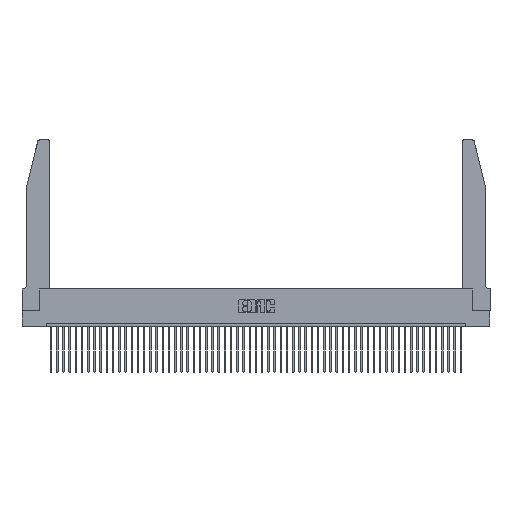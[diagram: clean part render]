
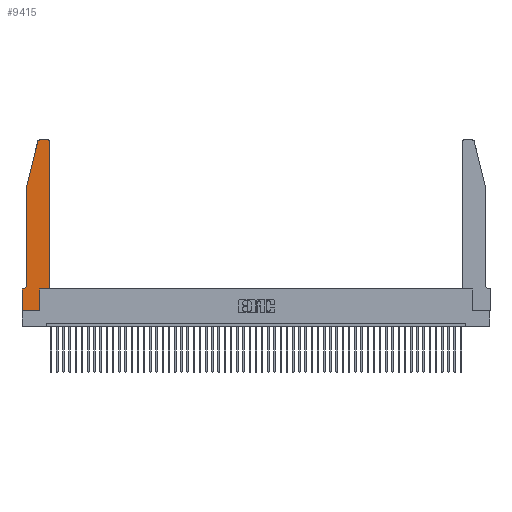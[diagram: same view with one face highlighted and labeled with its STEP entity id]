
A CAD part, top view. The second image highlights one B-rep face of the part: STEP entity #9415.
In plain terms, the highlighted planar face has unit normal (0, 0, 1).
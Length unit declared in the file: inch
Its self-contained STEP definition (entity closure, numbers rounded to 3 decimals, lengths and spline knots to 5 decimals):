
#374 = LINE ( 'NONE', #10518, #41643 ) ;
#1106 = VECTOR ( 'NONE', #31325, 39.37008 ) ;
#1204 = LINE ( 'NONE', #6719, #50765 ) ;
#2429 = CARTESIAN_POINT ( 'NONE',  ( 0.0755, 2., 0.37 ) ) ;
#2513 = ORIENTED_EDGE ( 'NONE', *, *, #3123, .T. ) ;
#2647 = EDGE_CURVE ( 'NONE', #16908, #18921, #16390, .T. ) ;
#2677 = EDGE_CURVE ( 'NONE', #35135, #7673, #44608, .T. ) ;
#3123 = EDGE_CURVE ( 'NONE', #8637, #47665, #18210, .T. ) ;
#3977 = CARTESIAN_POINT ( 'NONE',  ( 0., 0., 0.37 ) ) ;
#4345 = VERTEX_POINT ( 'NONE', #3977 ) ;
#4690 = EDGE_CURVE ( 'NONE', #18921, #37646, #39350, .T. ) ;
#5635 = CARTESIAN_POINT ( 'NONE',  ( 0.4505, 0.35, 0.37 ) ) ;
#5920 = EDGE_CURVE ( 'NONE', #7673, #25662, #12362, .T. ) ;
#6370 = DIRECTION ( 'NONE',  ( -1., 0., 0. ) ) ;
#6393 = EDGE_CURVE ( 'NONE', #35458, #16908, #32844, .T. ) ;
#6719 = CARTESIAN_POINT ( 'NONE',  ( 0.2605, 2.75, 0.37 ) ) ;
#7445 = PLANE ( 'NONE',  #38423 ) ;
#7526 = ORIENTED_EDGE ( 'NONE', *, *, #4690, .T. ) ;
#7673 = VERTEX_POINT ( 'NONE', #41694 ) ;
#7731 = VECTOR ( 'NONE', #43276, 39.37008 ) ;
#7817 = DIRECTION ( 'NONE',  ( 1., 0., 0. ) ) ;
#8637 = VERTEX_POINT ( 'NONE', #9405 ) ;
#9405 = CARTESIAN_POINT ( 'NONE',  ( 0.4505, 2.72, 0.37 ) ) ;
#9415 = ADVANCED_FACE ( 'NONE', ( #12563 ), #7445, .T. ) ;
#10518 = CARTESIAN_POINT ( 'NONE',  ( 0.0755, 0.35, 0.37 ) ) ;
#10722 = DIRECTION ( 'NONE',  ( 1., 0., 0. ) ) ;
#12362 = LINE ( 'NONE', #39153, #47496 ) ;
#12563 = FACE_OUTER_BOUND ( 'NONE', #18466, .T. ) ;
#13624 = CARTESIAN_POINT ( 'NONE',  ( 0.0755, 0.42, 0.37 ) ) ;
#14068 = AXIS2_PLACEMENT_3D ( 'NONE', #38728, #31158, #18724 ) ;
#14349 = DIRECTION ( 'NONE',  ( -1., 0., 0. ) ) ;
#14564 = CARTESIAN_POINT ( 'NONE',  ( 0., 0.35, 0.37 ) ) ;
#15141 = CARTESIAN_POINT ( 'NONE',  ( 0.284, 2.72, 0.37 ) ) ;
#15392 = VECTOR ( 'NONE', #33100, 39.37008 ) ;
#15919 = ORIENTED_EDGE ( 'NONE', *, *, #20522, .T. ) ;
#16390 = LINE ( 'NONE', #39221, #7731 ) ;
#16908 = VERTEX_POINT ( 'NONE', #48533 ) ;
#17867 = EDGE_CURVE ( 'NONE', #47665, #35458, #1204, .T. ) ;
#18210 = CIRCLE ( 'NONE', #14068, 0.03 ) ;
#18466 = EDGE_LOOP ( 'NONE', ( #30757, #20926, #44212, #7526, #37136, #26081, #39527, #15919, #37426, #43944, #51509, #2513 ) ) ;
#18724 = DIRECTION ( 'NONE',  ( 1., 0., 0. ) ) ;
#18921 = VERTEX_POINT ( 'NONE', #26406 ) ;
#19129 = DIRECTION ( 'NONE',  ( 1., 0., 0. ) ) ;
#19194 = CARTESIAN_POINT ( 'NONE',  ( 0.2865, 0., 0.37 ) ) ;
#19353 = VERTEX_POINT ( 'NONE', #50166 ) ;
#20522 = EDGE_CURVE ( 'NONE', #4345, #35135, #46096, .T. ) ;
#20926 = ORIENTED_EDGE ( 'NONE', *, *, #6393, .T. ) ;
#22070 = AXIS2_PLACEMENT_3D ( 'NONE', #39352, #30908, #39514 ) ;
#22544 = CARTESIAN_POINT ( 'NONE',  ( 0.4505, 0.35, 0.37 ) ) ;
#22667 = VECTOR ( 'NONE', #26216, 39.37008 ) ;
#23371 = VECTOR ( 'NONE', #35500, 39.37008 ) ;
#23710 = DIRECTION ( 'NONE',  ( 0., 0., 1. ) ) ;
#24046 = VECTOR ( 'NONE', #24860, 39.37008 ) ;
#24351 = VERTEX_POINT ( 'NONE', #49802 ) ;
#24860 = DIRECTION ( 'NONE',  ( 0., -1., 0. ) ) ;
#25662 = VERTEX_POINT ( 'NONE', #5635 ) ;
#26081 = ORIENTED_EDGE ( 'NONE', *, *, #37822, .T. ) ;
#26216 = DIRECTION ( 'NONE',  ( 0., 1., 0. ) ) ;
#26406 = CARTESIAN_POINT ( 'NONE',  ( 0.0755, 2., 0.37 ) ) ;
#29647 = CARTESIAN_POINT ( 'NONE',  ( 0., 0., 0.37 ) ) ;
#30581 = AXIS2_PLACEMENT_3D ( 'NONE', #15141, #23710, #7817 ) ;
#30757 = ORIENTED_EDGE ( 'NONE', *, *, #17867, .T. ) ;
#30908 = DIRECTION ( 'NONE',  ( 0., 0., -1. ) ) ;
#31140 = DIRECTION ( 'NONE',  ( 0., 0., 1. ) ) ;
#31158 = DIRECTION ( 'NONE',  ( 0., 0., 1. ) ) ;
#31325 = DIRECTION ( 'NONE',  ( 0., -1., 0. ) ) ;
#32844 = CIRCLE ( 'NONE', #30581, 0.03 ) ;
#33100 = DIRECTION ( 'NONE',  ( 1., 0., 0. ) ) ;
#33186 = CARTESIAN_POINT ( 'NONE',  ( 0.284, 2.75, 0.37 ) ) ;
#35135 = VERTEX_POINT ( 'NONE', #19194 ) ;
#35239 = EDGE_CURVE ( 'NONE', #37646, #19353, #35807, .T. ) ;
#35458 = VERTEX_POINT ( 'NONE', #33186 ) ;
#35500 = DIRECTION ( 'NONE',  ( 0., 1., 0. ) ) ;
#35807 = CIRCLE ( 'NONE', #22070, 0.07 ) ;
#36501 = LINE ( 'NONE', #48402, #24046 ) ;
#37136 = ORIENTED_EDGE ( 'NONE', *, *, #35239, .T. ) ;
#37426 = ORIENTED_EDGE ( 'NONE', *, *, #2677, .T. ) ;
#37646 = VERTEX_POINT ( 'NONE', #13624 ) ;
#37822 = EDGE_CURVE ( 'NONE', #19353, #24351, #374, .T. ) ;
#38423 = AXIS2_PLACEMENT_3D ( 'NONE', #14564, #31140, #10722 ) ;
#38728 = CARTESIAN_POINT ( 'NONE',  ( 0.4205, 2.72, 0.37 ) ) ;
#39153 = CARTESIAN_POINT ( 'NONE',  ( 0.4505, 0.35, 0.37 ) ) ;
#39221 = CARTESIAN_POINT ( 'NONE',  ( 0.0755, 2., 0.37 ) ) ;
#39350 = LINE ( 'NONE', #2429, #1106 ) ;
#39352 = CARTESIAN_POINT ( 'NONE',  ( 0.0055, 0.42, 0.37 ) ) ;
#39514 = DIRECTION ( 'NONE',  ( -1., 0., 0. ) ) ;
#39527 = ORIENTED_EDGE ( 'NONE', *, *, #46847, .T. ) ;
#41643 = VECTOR ( 'NONE', #14349, 39.37008 ) ;
#41694 = CARTESIAN_POINT ( 'NONE',  ( 0.2865, 0.35, 0.37 ) ) ;
#43276 = DIRECTION ( 'NONE',  ( -0.239, -0.971, 0. ) ) ;
#43407 = LINE ( 'NONE', #22544, #22667 ) ;
#43944 = ORIENTED_EDGE ( 'NONE', *, *, #5920, .T. ) ;
#44212 = ORIENTED_EDGE ( 'NONE', *, *, #2647, .T. ) ;
#44608 = LINE ( 'NONE', #51708, #23371 ) ;
#45290 = CARTESIAN_POINT ( 'NONE',  ( 0.4205, 2.75, 0.37 ) ) ;
#46096 = LINE ( 'NONE', #29647, #15392 ) ;
#46847 = EDGE_CURVE ( 'NONE', #24351, #4345, #36501, .T. ) ;
#47496 = VECTOR ( 'NONE', #19129, 39.37008 ) ;
#47665 = VERTEX_POINT ( 'NONE', #45290 ) ;
#47731 = EDGE_CURVE ( 'NONE', #25662, #8637, #43407, .T. ) ;
#48402 = CARTESIAN_POINT ( 'NONE',  ( 0., 0., 0.37 ) ) ;
#48533 = CARTESIAN_POINT ( 'NONE',  ( 0.25487, 2.72718, 0.37 ) ) ;
#49802 = CARTESIAN_POINT ( 'NONE',  ( 0., 0.35, 0.37 ) ) ;
#50166 = CARTESIAN_POINT ( 'NONE',  ( 0.0055, 0.35, 0.37 ) ) ;
#50765 = VECTOR ( 'NONE', #6370, 39.37008 ) ;
#51509 = ORIENTED_EDGE ( 'NONE', *, *, #47731, .T. ) ;
#51708 = CARTESIAN_POINT ( 'NONE',  ( 0.2865, 0.35, 0.37 ) ) ;
